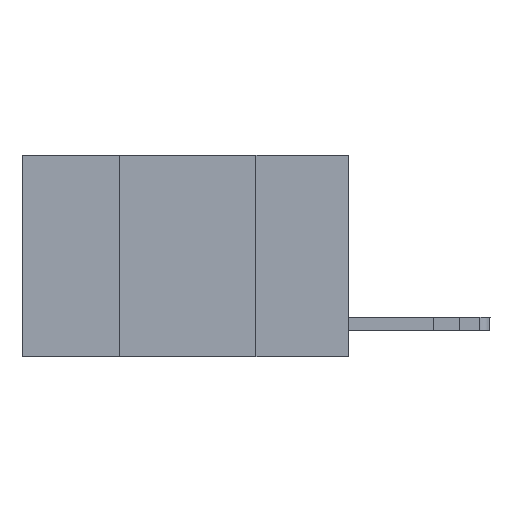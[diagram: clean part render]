
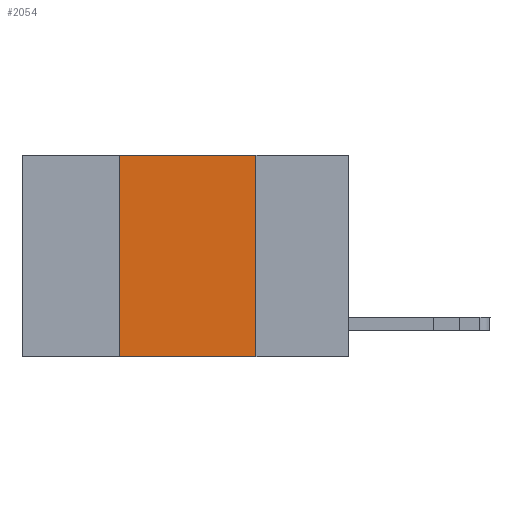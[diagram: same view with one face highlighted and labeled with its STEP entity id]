
A CAD part, left-side view. The second image highlights one B-rep face of the part: STEP entity #2054.
In plain terms, the highlighted planar face has unit normal (-1, 0, 0).
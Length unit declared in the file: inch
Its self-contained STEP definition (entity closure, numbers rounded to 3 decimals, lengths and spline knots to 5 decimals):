
#293 = CARTESIAN_POINT ( 'NONE',  ( 0., 0.17, -0.37 ) ) ;
#404 = VERTEX_POINT ( 'NONE', #725 ) ;
#725 = CARTESIAN_POINT ( 'NONE',  ( 0., 0.42, -0.37 ) ) ;
#1046 = EDGE_CURVE ( 'NONE', #9472, #5522, #15971, .T. ) ;
#1160 = LINE ( 'NONE', #10605, #8466 ) ;
#1385 = VECTOR ( 'NONE', #16913, 39.37008 ) ;
#2054 = ADVANCED_FACE ( 'NONE', ( #6800 ), #16223, .F. ) ;
#2111 = ORIENTED_EDGE ( 'NONE', *, *, #1046, .F. ) ;
#2314 = ORIENTED_EDGE ( 'NONE', *, *, #2945, .F. ) ;
#2352 = EDGE_CURVE ( 'NONE', #404, #16893, #2952, .T. ) ;
#2697 = EDGE_CURVE ( 'NONE', #404, #5522, #11837, .T. ) ;
#2707 = ORIENTED_EDGE ( 'NONE', *, *, #2352, .F. ) ;
#2945 = EDGE_CURVE ( 'NONE', #16893, #9472, #1160, .T. ) ;
#2952 = LINE ( 'NONE', #5226, #9741 ) ;
#3048 = ORIENTED_EDGE ( 'NONE', *, *, #2697, .T. ) ;
#5226 = CARTESIAN_POINT ( 'NONE',  ( 0., 0.42, 0. ) ) ;
#5325 = VECTOR ( 'NONE', #9980, 39.37008 ) ;
#5379 = DIRECTION ( 'NONE',  ( 0., 0., 1. ) ) ;
#5522 = VERTEX_POINT ( 'NONE', #293 ) ;
#6654 = EDGE_LOOP ( 'NONE', ( #2111, #2314, #2707, #3048 ) ) ;
#6800 = FACE_OUTER_BOUND ( 'NONE', #6654, .T. ) ;
#7113 = CARTESIAN_POINT ( 'NONE',  ( 0., 0.42, 0. ) ) ;
#7152 = CARTESIAN_POINT ( 'NONE',  ( 0., 0.17, 0. ) ) ;
#8466 = VECTOR ( 'NONE', #11144, 39.37008 ) ;
#9472 = VERTEX_POINT ( 'NONE', #7152 ) ;
#9486 = AXIS2_PLACEMENT_3D ( 'NONE', #16128, #16071, #16034 ) ;
#9741 = VECTOR ( 'NONE', #5379, 39.37008 ) ;
#9980 = DIRECTION ( 'NONE',  ( 0., 0., -1. ) ) ;
#10114 = CARTESIAN_POINT ( 'NONE',  ( 0., 0.17, 0. ) ) ;
#10605 = CARTESIAN_POINT ( 'NONE',  ( 0., 0.6, 0. ) ) ;
#11144 = DIRECTION ( 'NONE',  ( 0., -1., 0. ) ) ;
#11837 = LINE ( 'NONE', #17207, #1385 ) ;
#15971 = LINE ( 'NONE', #10114, #5325 ) ;
#16034 = DIRECTION ( 'NONE',  ( 0., 0., -1. ) ) ;
#16071 = DIRECTION ( 'NONE',  ( 1., 0., 0. ) ) ;
#16128 = CARTESIAN_POINT ( 'NONE',  ( 0., 0.6, 0. ) ) ;
#16223 = PLANE ( 'NONE',  #9486 ) ;
#16893 = VERTEX_POINT ( 'NONE', #7113 ) ;
#16913 = DIRECTION ( 'NONE',  ( 0., -1., 0. ) ) ;
#17207 = CARTESIAN_POINT ( 'NONE',  ( 0., 0.6, -0.37 ) ) ;
